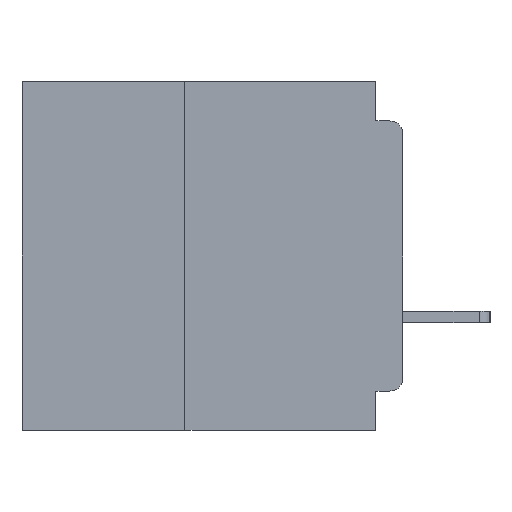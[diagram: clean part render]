
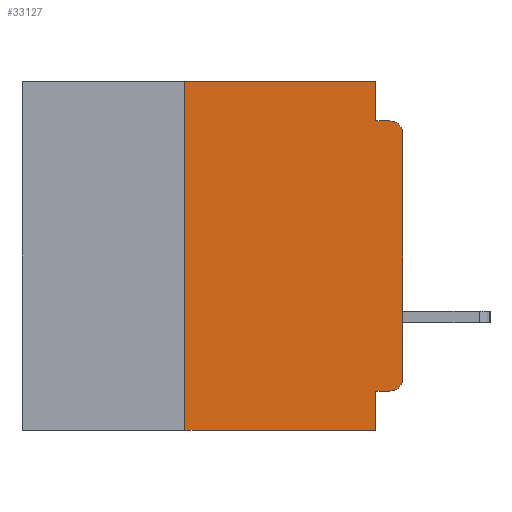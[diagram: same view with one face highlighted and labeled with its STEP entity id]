
A CAD part, left-side view. The second image highlights one B-rep face of the part: STEP entity #33127.
In plain terms, the highlighted planar face has unit normal (-1, 0, 0).
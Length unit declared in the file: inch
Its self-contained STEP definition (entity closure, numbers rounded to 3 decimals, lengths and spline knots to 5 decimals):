
#707 = DIRECTION ( 'NONE',  ( 0., 0., -1. ) ) ;
#1046 = ORIENTED_EDGE ( 'NONE', *, *, #30491, .T. ) ;
#1405 = LINE ( 'NONE', #12192, #24659 ) ;
#1597 = VERTEX_POINT ( 'NONE', #13218 ) ;
#1651 = VERTEX_POINT ( 'NONE', #14668 ) ;
#1951 = CARTESIAN_POINT ( 'NONE',  ( 0., 0.015, -0.045 ) ) ;
#2428 = LINE ( 'NONE', #16488, #9835 ) ;
#2556 = DIRECTION ( 'NONE',  ( 0., 0., -1. ) ) ;
#2737 = LINE ( 'NONE', #25519, #34089 ) ;
#3828 = DIRECTION ( 'NONE',  ( 0., 0., -1. ) ) ;
#4517 = VERTEX_POINT ( 'NONE', #12117 ) ;
#4703 = CARTESIAN_POINT ( 'NONE',  ( 0., 0.031, 0. ) ) ;
#5187 = LINE ( 'NONE', #12824, #20020 ) ;
#6602 = DIRECTION ( 'NONE',  ( -1., 0., 0. ) ) ;
#6652 = AXIS2_PLACEMENT_3D ( 'NONE', #6838, #22735, #3828 ) ;
#6838 = CARTESIAN_POINT ( 'NONE',  ( 0., 0.437, 0. ) ) ;
#7961 = VECTOR ( 'NONE', #18052, 39.37008 ) ;
#8114 = CARTESIAN_POINT ( 'NONE',  ( 0., 0.031, -0.4 ) ) ;
#8294 = VERTEX_POINT ( 'NONE', #8114 ) ;
#8520 = CARTESIAN_POINT ( 'NONE',  ( 0., 0.437, -0.4 ) ) ;
#9835 = VECTOR ( 'NONE', #707, 39.37008 ) ;
#10023 = ORIENTED_EDGE ( 'NONE', *, *, #35355, .F. ) ;
#11662 = EDGE_CURVE ( 'NONE', #13913, #31825, #16262, .T. ) ;
#12040 = AXIS2_PLACEMENT_3D ( 'NONE', #25540, #6602, #28639 ) ;
#12117 = CARTESIAN_POINT ( 'NONE',  ( 0., 0.031, -0.355 ) ) ;
#12126 = CARTESIAN_POINT ( 'NONE',  ( 0., 0.437, 0. ) ) ;
#12192 = CARTESIAN_POINT ( 'NONE',  ( 0., 0.031, 0. ) ) ;
#12210 = CIRCLE ( 'NONE', #12040, 0.015 ) ;
#12824 = CARTESIAN_POINT ( 'NONE',  ( 0., 0., -0.045 ) ) ;
#12977 = ORIENTED_EDGE ( 'NONE', *, *, #13708, .F. ) ;
#13218 = CARTESIAN_POINT ( 'NONE',  ( 0., 0.031, -0.045 ) ) ;
#13232 = DIRECTION ( 'NONE',  ( 0., 0., 1. ) ) ;
#13708 = EDGE_CURVE ( 'NONE', #1597, #36777, #5187, .T. ) ;
#13913 = VERTEX_POINT ( 'NONE', #32630 ) ;
#14551 = CIRCLE ( 'NONE', #30759, 0.015 ) ;
#14668 = CARTESIAN_POINT ( 'NONE',  ( 0., 0.25, -0.4 ) ) ;
#15329 = DIRECTION ( 'NONE',  ( 0., -1., 0. ) ) ;
#15402 = DIRECTION ( 'NONE',  ( 0., 0., -1. ) ) ;
#16194 = CARTESIAN_POINT ( 'NONE',  ( 0., 0., -0.34 ) ) ;
#16262 = LINE ( 'NONE', #12126, #17234 ) ;
#16488 = CARTESIAN_POINT ( 'NONE',  ( 0., 0.031, -0.4 ) ) ;
#17234 = VECTOR ( 'NONE', #15329, 39.37008 ) ;
#17355 = LINE ( 'NONE', #8520, #7961 ) ;
#18052 = DIRECTION ( 'NONE',  ( 0., -1., 0. ) ) ;
#19564 = PLANE ( 'NONE',  #6652 ) ;
#20020 = VECTOR ( 'NONE', #25522, 39.37008 ) ;
#20400 = ORIENTED_EDGE ( 'NONE', *, *, #20824, .T. ) ;
#20675 = CARTESIAN_POINT ( 'NONE',  ( 0., 0., -0.06 ) ) ;
#20701 = LINE ( 'NONE', #31368, #36187 ) ;
#20824 = EDGE_CURVE ( 'NONE', #27954, #21686, #14551, .T. ) ;
#21286 = VECTOR ( 'NONE', #13232, 39.37008 ) ;
#21461 = DIRECTION ( 'NONE',  ( -1., 0., 0. ) ) ;
#21686 = VERTEX_POINT ( 'NONE', #16194 ) ;
#22362 = ORIENTED_EDGE ( 'NONE', *, *, #11662, .F. ) ;
#22735 = DIRECTION ( 'NONE',  ( 1., 0., 0. ) ) ;
#22834 = ORIENTED_EDGE ( 'NONE', *, *, #27147, .T. ) ;
#24271 = LINE ( 'NONE', #25913, #21286 ) ;
#24659 = VECTOR ( 'NONE', #15402, 39.37008 ) ;
#24841 = ORIENTED_EDGE ( 'NONE', *, *, #26086, .F. ) ;
#24870 = FACE_OUTER_BOUND ( 'NONE', #32616, .T. ) ;
#25519 = CARTESIAN_POINT ( 'NONE',  ( 0., 0.25, -0.4 ) ) ;
#25522 = DIRECTION ( 'NONE',  ( 0., -1., 0. ) ) ;
#25540 = CARTESIAN_POINT ( 'NONE',  ( 0., 0.015, -0.06 ) ) ;
#25913 = CARTESIAN_POINT ( 'NONE',  ( 0., 0., 0. ) ) ;
#26086 = EDGE_CURVE ( 'NONE', #4517, #8294, #2428, .T. ) ;
#26280 = ORIENTED_EDGE ( 'NONE', *, *, #30201, .T. ) ;
#26417 = CARTESIAN_POINT ( 'NONE',  ( 0., 0.015, -0.355 ) ) ;
#27147 = EDGE_CURVE ( 'NONE', #29228, #36777, #12210, .T. ) ;
#27954 = VERTEX_POINT ( 'NONE', #26417 ) ;
#28639 = DIRECTION ( 'NONE',  ( 0., 0., -1. ) ) ;
#28742 = DIRECTION ( 'NONE',  ( 0., 0., 1. ) ) ;
#29228 = VERTEX_POINT ( 'NONE', #20675 ) ;
#30201 = EDGE_CURVE ( 'NONE', #1651, #8294, #17355, .T. ) ;
#30491 = EDGE_CURVE ( 'NONE', #21686, #29228, #24271, .T. ) ;
#30759 = AXIS2_PLACEMENT_3D ( 'NONE', #39891, #21461, #2556 ) ;
#31368 = CARTESIAN_POINT ( 'NONE',  ( 0., 0., -0.355 ) ) ;
#31825 = VERTEX_POINT ( 'NONE', #4703 ) ;
#32264 = EDGE_CURVE ( 'NONE', #1651, #13913, #2737, .T. ) ;
#32616 = EDGE_LOOP ( 'NONE', ( #1046, #22834, #12977, #37774, #22362, #39668, #26280, #24841, #10023, #20400 ) ) ;
#32630 = CARTESIAN_POINT ( 'NONE',  ( 0., 0.25, 0. ) ) ;
#33127 = ADVANCED_FACE ( 'NONE', ( #24870 ), #19564, .F. ) ;
#34089 = VECTOR ( 'NONE', #28742, 39.37008 ) ;
#34453 = DIRECTION ( 'NONE',  ( 0., 1., 0. ) ) ;
#35355 = EDGE_CURVE ( 'NONE', #27954, #4517, #20701, .T. ) ;
#36187 = VECTOR ( 'NONE', #34453, 39.37008 ) ;
#36346 = EDGE_CURVE ( 'NONE', #31825, #1597, #1405, .T. ) ;
#36777 = VERTEX_POINT ( 'NONE', #1951 ) ;
#37774 = ORIENTED_EDGE ( 'NONE', *, *, #36346, .F. ) ;
#39668 = ORIENTED_EDGE ( 'NONE', *, *, #32264, .F. ) ;
#39891 = CARTESIAN_POINT ( 'NONE',  ( 0., 0.015, -0.34 ) ) ;
